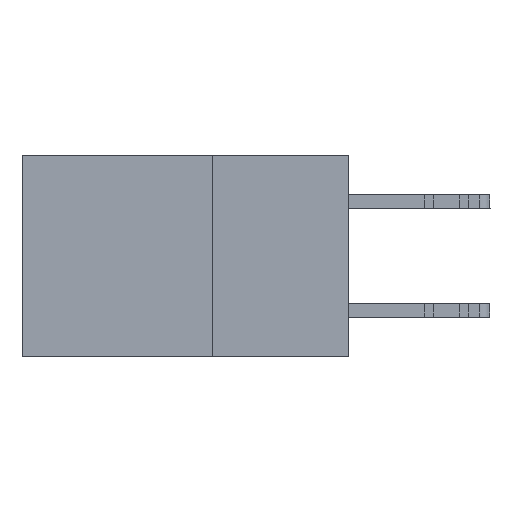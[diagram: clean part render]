
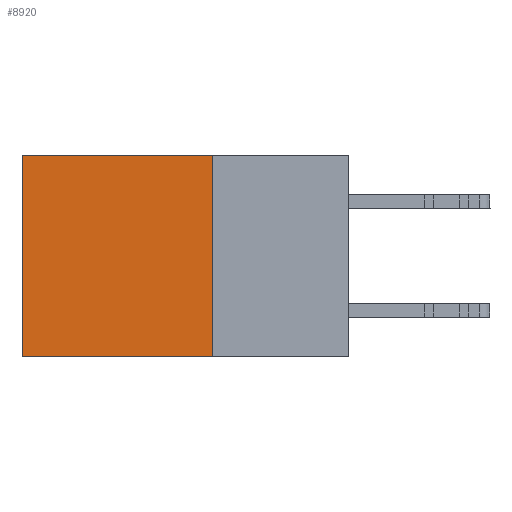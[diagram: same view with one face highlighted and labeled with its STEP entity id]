
A CAD part, left-side view. The second image highlights one B-rep face of the part: STEP entity #8920.
In plain terms, the highlighted planar face has unit normal (-1, 0, 0).
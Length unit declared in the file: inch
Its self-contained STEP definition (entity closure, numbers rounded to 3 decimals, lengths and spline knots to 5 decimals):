
#168 = PLANE ( 'NONE',  #7739 ) ;
#1541 = LINE ( 'NONE', #26543, #23080 ) ;
#2394 = VERTEX_POINT ( 'NONE', #14518 ) ;
#3182 = VERTEX_POINT ( 'NONE', #4321 ) ;
#3769 = DIRECTION ( 'NONE',  ( 0., 1., 0. ) ) ;
#3778 = LINE ( 'NONE', #8684, #19153 ) ;
#4321 = CARTESIAN_POINT ( 'NONE',  ( 0.2615, 0.25, 0. ) ) ;
#4387 = DIRECTION ( 'NONE',  ( 0., 0., -1. ) ) ;
#5283 = EDGE_CURVE ( 'NONE', #3182, #20429, #3778, .T. ) ;
#5322 = VECTOR ( 'NONE', #16713, 39.37008 ) ;
#5665 = ORIENTED_EDGE ( 'NONE', *, *, #7431, .F. ) ;
#6881 = CARTESIAN_POINT ( 'NONE',  ( 0.2615, 0.6, -0.37 ) ) ;
#7431 = EDGE_CURVE ( 'NONE', #3182, #2394, #12176, .T. ) ;
#7739 = AXIS2_PLACEMENT_3D ( 'NONE', #14814, #16909, #4387 ) ;
#8106 = LINE ( 'NONE', #6881, #18524 ) ;
#8202 = FACE_OUTER_BOUND ( 'NONE', #13441, .T. ) ;
#8367 = CARTESIAN_POINT ( 'NONE',  ( 0.2615, 0.25, -0.37 ) ) ;
#8684 = CARTESIAN_POINT ( 'NONE',  ( 0.2615, 0.25, 0. ) ) ;
#8851 = ORIENTED_EDGE ( 'NONE', *, *, #18333, .T. ) ;
#8920 = ADVANCED_FACE ( 'NONE', ( #8202 ), #168, .F. ) ;
#10130 = EDGE_CURVE ( 'NONE', #2394, #18678, #1541, .T. ) ;
#11080 = DIRECTION ( 'NONE',  ( 0., 0., -1. ) ) ;
#12176 = LINE ( 'NONE', #8367, #5322 ) ;
#13441 = EDGE_LOOP ( 'NONE', ( #8851, #24867, #5665, #18006 ) ) ;
#14244 = CARTESIAN_POINT ( 'NONE',  ( 0.2615, 0.6, -0.37 ) ) ;
#14518 = CARTESIAN_POINT ( 'NONE',  ( 0.2615, 0.25, -0.37 ) ) ;
#14814 = CARTESIAN_POINT ( 'NONE',  ( 0.2615, 0.25, -0.37 ) ) ;
#16713 = DIRECTION ( 'NONE',  ( 0., 0., -1. ) ) ;
#16909 = DIRECTION ( 'NONE',  ( 1., 0., 0. ) ) ;
#17022 = DIRECTION ( 'NONE',  ( 0., 1., 0. ) ) ;
#18006 = ORIENTED_EDGE ( 'NONE', *, *, #5283, .T. ) ;
#18333 = EDGE_CURVE ( 'NONE', #20429, #18678, #8106, .T. ) ;
#18524 = VECTOR ( 'NONE', #11080, 39.37008 ) ;
#18678 = VERTEX_POINT ( 'NONE', #14244 ) ;
#19153 = VECTOR ( 'NONE', #17022, 39.37008 ) ;
#20429 = VERTEX_POINT ( 'NONE', #25499 ) ;
#23080 = VECTOR ( 'NONE', #3769, 39.37008 ) ;
#24867 = ORIENTED_EDGE ( 'NONE', *, *, #10130, .F. ) ;
#25499 = CARTESIAN_POINT ( 'NONE',  ( 0.2615, 0.6, 0. ) ) ;
#26543 = CARTESIAN_POINT ( 'NONE',  ( 0.2615, 0.25, -0.37 ) ) ;
